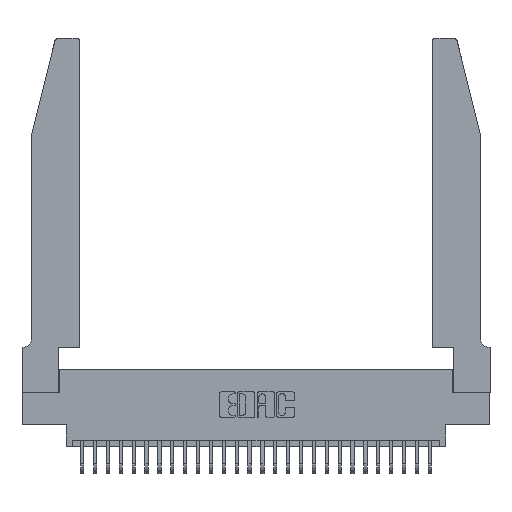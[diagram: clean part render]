
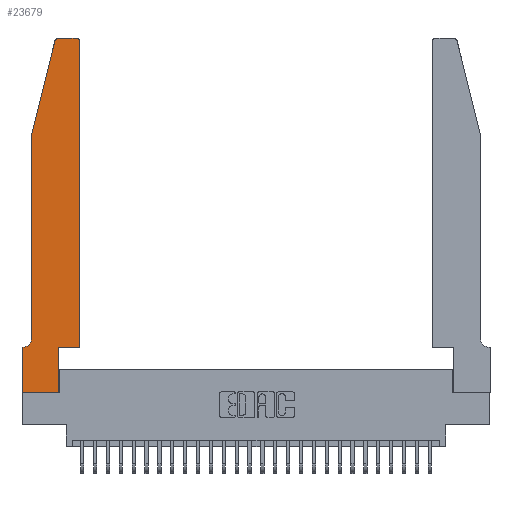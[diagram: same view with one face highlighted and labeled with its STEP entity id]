
A CAD part, top view. The second image highlights one B-rep face of the part: STEP entity #23679.
In plain terms, the highlighted planar face has unit normal (0, 0, 1).
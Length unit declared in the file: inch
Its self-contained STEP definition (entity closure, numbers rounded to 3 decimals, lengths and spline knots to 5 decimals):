
#151 = DIRECTION ( 'NONE',  ( -1., 0., 0. ) ) ;
#510 = VECTOR ( 'NONE', #1432, 39.37008 ) ;
#700 = VERTEX_POINT ( 'NONE', #24300 ) ;
#850 = VERTEX_POINT ( 'NONE', #16033 ) ;
#1262 = CARTESIAN_POINT ( 'NONE',  ( 0.4505, 0.35, 0.37 ) ) ;
#1432 = DIRECTION ( 'NONE',  ( 1., 0., 0. ) ) ;
#1575 = ORIENTED_EDGE ( 'NONE', *, *, #8863, .T. ) ;
#1885 = ORIENTED_EDGE ( 'NONE', *, *, #16023, .T. ) ;
#2029 = VERTEX_POINT ( 'NONE', #26544 ) ;
#2231 = EDGE_LOOP ( 'NONE', ( #16732, #1885, #5686, #4625, #1575, #11847, #27844, #6659, #9518, #19776, #23002, #19086 ) ) ;
#2340 = CARTESIAN_POINT ( 'NONE',  ( 0.284, 2.72, 0.37 ) ) ;
#2501 = VERTEX_POINT ( 'NONE', #14798 ) ;
#3137 = CARTESIAN_POINT ( 'NONE',  ( 0.0755, 2., 0.37 ) ) ;
#3514 = CARTESIAN_POINT ( 'NONE',  ( 0.0055, 0.42, 0.37 ) ) ;
#4155 = VECTOR ( 'NONE', #151, 39.37008 ) ;
#4497 = CARTESIAN_POINT ( 'NONE',  ( 0., 0., 0.37 ) ) ;
#4625 = ORIENTED_EDGE ( 'NONE', *, *, #26608, .T. ) ;
#4770 = DIRECTION ( 'NONE',  ( 1., 0., 0. ) ) ;
#5021 = EDGE_CURVE ( 'NONE', #15385, #14976, #24788, .T. ) ;
#5120 = EDGE_CURVE ( 'NONE', #25293, #18547, #11798, .T. ) ;
#5484 = CARTESIAN_POINT ( 'NONE',  ( 0.2865, 0.35, 0.37 ) ) ;
#5594 = DIRECTION ( 'NONE',  ( -0.239, -0.971, 0. ) ) ;
#5686 = ORIENTED_EDGE ( 'NONE', *, *, #19391, .T. ) ;
#5980 = DIRECTION ( 'NONE',  ( -1., 0., 0. ) ) ;
#6424 = EDGE_CURVE ( 'NONE', #14976, #29891, #12539, .T. ) ;
#6596 = CARTESIAN_POINT ( 'NONE',  ( 0.0755, 0.42, 0.37 ) ) ;
#6659 = ORIENTED_EDGE ( 'NONE', *, *, #5021, .T. ) ;
#7107 = CARTESIAN_POINT ( 'NONE',  ( 0.0055, 0.35, 0.37 ) ) ;
#7941 = DIRECTION ( 'NONE',  ( 0., 1., 0. ) ) ;
#8022 = CARTESIAN_POINT ( 'NONE',  ( 0., 0., 0.37 ) ) ;
#8205 = CARTESIAN_POINT ( 'NONE',  ( 0.4505, 0.35, 0.37 ) ) ;
#8385 = EDGE_CURVE ( 'NONE', #29469, #850, #10973, .T. ) ;
#8671 = EDGE_CURVE ( 'NONE', #18547, #12661, #17452, .T. ) ;
#8863 = EDGE_CURVE ( 'NONE', #20237, #29469, #17084, .T. ) ;
#9138 = LINE ( 'NONE', #1262, #20736 ) ;
#9518 = ORIENTED_EDGE ( 'NONE', *, *, #6424, .T. ) ;
#10263 = DIRECTION ( 'NONE',  ( 0., 0., 1. ) ) ;
#10264 = VECTOR ( 'NONE', #24559, 39.37008 ) ;
#10553 = LINE ( 'NONE', #8022, #16682 ) ;
#10973 = LINE ( 'NONE', #13063, #10264 ) ;
#11345 = DIRECTION ( 'NONE',  ( 0., 0., 1. ) ) ;
#11798 = CIRCLE ( 'NONE', #14873, 0.03 ) ;
#11847 = ORIENTED_EDGE ( 'NONE', *, *, #8385, .T. ) ;
#11940 = CARTESIAN_POINT ( 'NONE',  ( 0.0755, 2., 0.37 ) ) ;
#12088 = VECTOR ( 'NONE', #17446, 39.37008 ) ;
#12095 = LINE ( 'NONE', #3137, #21489 ) ;
#12293 = CARTESIAN_POINT ( 'NONE',  ( 0.4505, 2.72, 0.37 ) ) ;
#12371 = AXIS2_PLACEMENT_3D ( 'NONE', #3514, #20006, #5980 ) ;
#12539 = LINE ( 'NONE', #5484, #24086 ) ;
#12661 = VERTEX_POINT ( 'NONE', #18591 ) ;
#12795 = AXIS2_PLACEMENT_3D ( 'NONE', #24069, #10263, #26437 ) ;
#13035 = EDGE_CURVE ( 'NONE', #2501, #25293, #24342, .T. ) ;
#13063 = CARTESIAN_POINT ( 'NONE',  ( 0.0755, 0.35, 0.37 ) ) ;
#13132 = EDGE_CURVE ( 'NONE', #29891, #2501, #9138, .T. ) ;
#13362 = CARTESIAN_POINT ( 'NONE',  ( 0.2865, 0.35, 0.37 ) ) ;
#14796 = PLANE ( 'NONE',  #12795 ) ;
#14798 = CARTESIAN_POINT ( 'NONE',  ( 0.4505, 0.35, 0.37 ) ) ;
#14873 = AXIS2_PLACEMENT_3D ( 'NONE', #25156, #11345, #27519 ) ;
#14976 = VERTEX_POINT ( 'NONE', #24077 ) ;
#15058 = LINE ( 'NONE', #11940, #27355 ) ;
#15385 = VERTEX_POINT ( 'NONE', #4497 ) ;
#15679 = CARTESIAN_POINT ( 'NONE',  ( 0., 0., 0.37 ) ) ;
#16023 = EDGE_CURVE ( 'NONE', #12661, #2029, #17653, .T. ) ;
#16033 = CARTESIAN_POINT ( 'NONE',  ( 0., 0.35, 0.37 ) ) ;
#16682 = VECTOR ( 'NONE', #28809, 39.37008 ) ;
#16732 = ORIENTED_EDGE ( 'NONE', *, *, #8671, .T. ) ;
#17084 = CIRCLE ( 'NONE', #12371, 0.07 ) ;
#17446 = DIRECTION ( 'NONE',  ( 0., 1., 0. ) ) ;
#17452 = LINE ( 'NONE', #28316, #4155 ) ;
#17653 = CIRCLE ( 'NONE', #23482, 0.03 ) ;
#18547 = VERTEX_POINT ( 'NONE', #30302 ) ;
#18591 = CARTESIAN_POINT ( 'NONE',  ( 0.284, 2.75, 0.37 ) ) ;
#18889 = DIRECTION ( 'NONE',  ( 0., 0., 1. ) ) ;
#19086 = ORIENTED_EDGE ( 'NONE', *, *, #5120, .T. ) ;
#19391 = EDGE_CURVE ( 'NONE', #2029, #700, #12095, .T. ) ;
#19776 = ORIENTED_EDGE ( 'NONE', *, *, #13132, .T. ) ;
#20006 = DIRECTION ( 'NONE',  ( 0., 0., -1. ) ) ;
#20237 = VERTEX_POINT ( 'NONE', #6596 ) ;
#20736 = VECTOR ( 'NONE', #24702, 39.37008 ) ;
#21489 = VECTOR ( 'NONE', #5594, 39.37008 ) ;
#23002 = ORIENTED_EDGE ( 'NONE', *, *, #13035, .T. ) ;
#23482 = AXIS2_PLACEMENT_3D ( 'NONE', #2340, #18889, #4770 ) ;
#23679 = ADVANCED_FACE ( 'NONE', ( #30315 ), #14796, .T. ) ;
#24069 = CARTESIAN_POINT ( 'NONE',  ( 0., 0.35, 0.37 ) ) ;
#24077 = CARTESIAN_POINT ( 'NONE',  ( 0.2865, 0., 0.37 ) ) ;
#24086 = VECTOR ( 'NONE', #7941, 39.37008 ) ;
#24300 = CARTESIAN_POINT ( 'NONE',  ( 0.0755, 2., 0.37 ) ) ;
#24342 = LINE ( 'NONE', #8205, #12088 ) ;
#24559 = DIRECTION ( 'NONE',  ( -1., 0., 0. ) ) ;
#24702 = DIRECTION ( 'NONE',  ( 1., 0., 0. ) ) ;
#24788 = LINE ( 'NONE', #15679, #510 ) ;
#25156 = CARTESIAN_POINT ( 'NONE',  ( 0.4205, 2.72, 0.37 ) ) ;
#25293 = VERTEX_POINT ( 'NONE', #12293 ) ;
#26437 = DIRECTION ( 'NONE',  ( 1., 0., 0. ) ) ;
#26544 = CARTESIAN_POINT ( 'NONE',  ( 0.25487, 2.72718, 0.37 ) ) ;
#26608 = EDGE_CURVE ( 'NONE', #700, #20237, #15058, .T. ) ;
#27355 = VECTOR ( 'NONE', #28205, 39.37008 ) ;
#27519 = DIRECTION ( 'NONE',  ( 1., 0., 0. ) ) ;
#27844 = ORIENTED_EDGE ( 'NONE', *, *, #30252, .T. ) ;
#28205 = DIRECTION ( 'NONE',  ( 0., -1., 0. ) ) ;
#28316 = CARTESIAN_POINT ( 'NONE',  ( 0.2605, 2.75, 0.37 ) ) ;
#28809 = DIRECTION ( 'NONE',  ( 0., -1., 0. ) ) ;
#29469 = VERTEX_POINT ( 'NONE', #7107 ) ;
#29891 = VERTEX_POINT ( 'NONE', #13362 ) ;
#30252 = EDGE_CURVE ( 'NONE', #850, #15385, #10553, .T. ) ;
#30302 = CARTESIAN_POINT ( 'NONE',  ( 0.4205, 2.75, 0.37 ) ) ;
#30315 = FACE_OUTER_BOUND ( 'NONE', #2231, .T. ) ;
